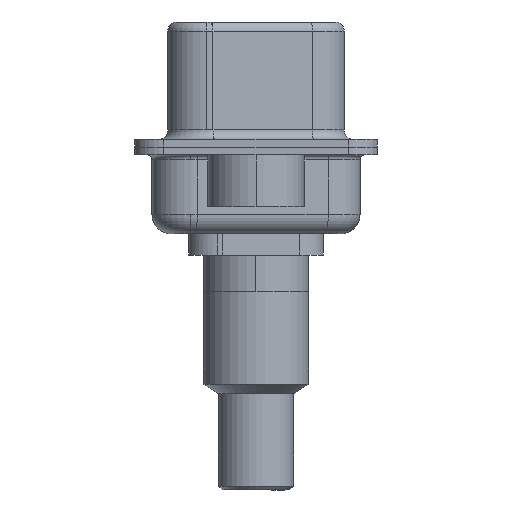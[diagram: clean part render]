
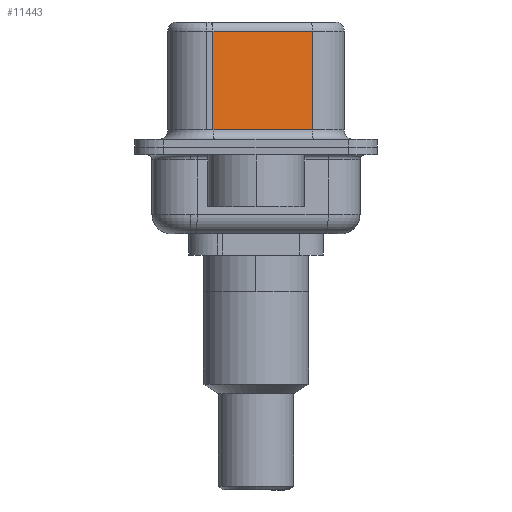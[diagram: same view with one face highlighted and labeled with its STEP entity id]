
A CAD part, left-side view. The second image highlights one B-rep face of the part: STEP entity #11443.
In plain terms, the highlighted planar face has unit normal (-0.985, -0.174, 0).
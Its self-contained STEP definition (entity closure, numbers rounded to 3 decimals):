
#25 = ORIENTED_EDGE ( 'NONE', *, *, #16427, .T. ) ;
#824 = EDGE_CURVE ( 'NONE', #14209, #17362, #23172, .T. ) ;
#1302 = LINE ( 'NONE', #13095, #7013 ) ;
#1440 = VERTEX_POINT ( 'NONE', #2078 ) ;
#1856 = EDGE_LOOP ( 'NONE', ( #7976, #5363, #25, #18399 ) ) ;
#2078 = CARTESIAN_POINT ( 'NONE',  ( 3.67, 2.233, 6.02 ) ) ;
#2591 = EDGE_CURVE ( 'NONE', #15288, #17362, #1302, .T. ) ;
#3407 = VECTOR ( 'NONE', #18501, 1000. ) ;
#3431 = CARTESIAN_POINT ( 'NONE',  ( 3.67, 2.233, 0.9 ) ) ;
#3503 = DIRECTION ( 'NONE',  ( -0.174, 0.985, 0. ) ) ;
#4229 = LINE ( 'NONE', #5834, #18903 ) ;
#5007 = CARTESIAN_POINT ( 'NONE',  ( 4.58, -2.927, 0.9 ) ) ;
#5363 = ORIENTED_EDGE ( 'NONE', *, *, #18441, .T. ) ;
#5496 = CARTESIAN_POINT ( 'NONE',  ( 4.58, -2.927, 0.9 ) ) ;
#5834 = CARTESIAN_POINT ( 'NONE',  ( 4.58, -2.927, 6.02 ) ) ;
#7013 = VECTOR ( 'NONE', #16377, 1000. ) ;
#7976 = ORIENTED_EDGE ( 'NONE', *, *, #2591, .F. ) ;
#8848 = LINE ( 'NONE', #9789, #17806 ) ;
#9041 = AXIS2_PLACEMENT_3D ( 'NONE', #13034, #14951, #3503 ) ;
#9789 = CARTESIAN_POINT ( 'NONE',  ( 3.67, 2.233, 6.52 ) ) ;
#11443 = ADVANCED_FACE ( 'NONE', ( #21064 ), #24558, .F. ) ;
#11621 = DIRECTION ( 'NONE',  ( -0.174, 0.985, 0. ) ) ;
#13034 = CARTESIAN_POINT ( 'NONE',  ( 4.58, -2.927, 6.52 ) ) ;
#13095 = CARTESIAN_POINT ( 'NONE',  ( 4.58, -2.927, 6.52 ) ) ;
#14209 = VERTEX_POINT ( 'NONE', #3431 ) ;
#14951 = DIRECTION ( 'NONE',  ( 0.985, 0.174, 0. ) ) ;
#15288 = VERTEX_POINT ( 'NONE', #17934 ) ;
#16377 = DIRECTION ( 'NONE',  ( 0., 0., -1. ) ) ;
#16427 = EDGE_CURVE ( 'NONE', #1440, #14209, #8848, .T. ) ;
#17362 = VERTEX_POINT ( 'NONE', #5007 ) ;
#17484 = DIRECTION ( 'NONE',  ( 0., 0., -1. ) ) ;
#17806 = VECTOR ( 'NONE', #17484, 1000. ) ;
#17934 = CARTESIAN_POINT ( 'NONE',  ( 4.58, -2.927, 6.02 ) ) ;
#18399 = ORIENTED_EDGE ( 'NONE', *, *, #824, .T. ) ;
#18441 = EDGE_CURVE ( 'NONE', #15288, #1440, #4229, .T. ) ;
#18501 = DIRECTION ( 'NONE',  ( 0.174, -0.985, 0. ) ) ;
#18903 = VECTOR ( 'NONE', #11621, 1000. ) ;
#21064 = FACE_OUTER_BOUND ( 'NONE', #1856, .T. ) ;
#23172 = LINE ( 'NONE', #5496, #3407 ) ;
#24558 = PLANE ( 'NONE',  #9041 ) ;
